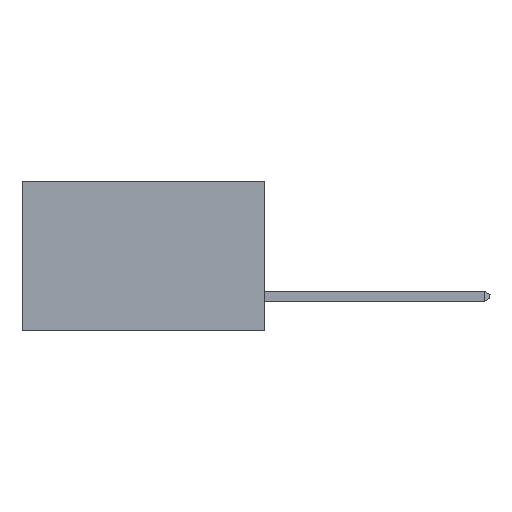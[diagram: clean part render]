
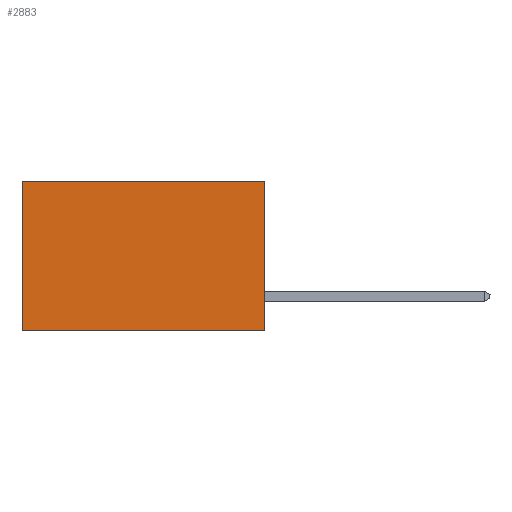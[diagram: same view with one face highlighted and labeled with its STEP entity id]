
A CAD part, left-side view. The second image highlights one B-rep face of the part: STEP entity #2883.
In plain terms, the highlighted planar face has unit normal (-1, 0, 0).
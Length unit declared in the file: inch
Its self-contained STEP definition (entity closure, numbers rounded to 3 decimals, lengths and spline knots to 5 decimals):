
#485 = DIRECTION ( 'NONE',  ( 0., 0., -1. ) ) ;
#1807 = ORIENTED_EDGE ( 'NONE', *, *, #14942, .F. ) ;
#2088 = VERTEX_POINT ( 'NONE', #3233 ) ;
#2535 = CARTESIAN_POINT ( 'NONE',  ( 0.298, 0.6, -0.37 ) ) ;
#2547 = PLANE ( 'NONE',  #7982 ) ;
#2594 = DIRECTION ( 'NONE',  ( 1., 0., 0. ) ) ;
#2863 = LINE ( 'NONE', #11257, #3268 ) ;
#2883 = ADVANCED_FACE ( 'NONE', ( #11976 ), #2547, .F. ) ;
#3084 = CARTESIAN_POINT ( 'NONE',  ( 0.298, 0.6, 0. ) ) ;
#3133 = LINE ( 'NONE', #15592, #11950 ) ;
#3140 = CARTESIAN_POINT ( 'NONE',  ( 0.298, 0.6, 0. ) ) ;
#3233 = CARTESIAN_POINT ( 'NONE',  ( 0.298, 0., 0. ) ) ;
#3268 = VECTOR ( 'NONE', #11429, 39.37008 ) ;
#3695 = DIRECTION ( 'NONE',  ( 0., 1., 0. ) ) ;
#3836 = LINE ( 'NONE', #3084, #4209 ) ;
#4209 = VECTOR ( 'NONE', #485, 39.37008 ) ;
#4692 = DIRECTION ( 'NONE',  ( 0., 0., -1. ) ) ;
#4791 = CARTESIAN_POINT ( 'NONE',  ( 0.298, 0., 0. ) ) ;
#5003 = VERTEX_POINT ( 'NONE', #13782 ) ;
#6920 = ORIENTED_EDGE ( 'NONE', *, *, #10507, .T. ) ;
#7278 = DIRECTION ( 'NONE',  ( 0., 0., -1. ) ) ;
#7982 = AXIS2_PLACEMENT_3D ( 'NONE', #13383, #2594, #7278 ) ;
#9588 = ORIENTED_EDGE ( 'NONE', *, *, #11350, .F. ) ;
#10507 = EDGE_CURVE ( 'NONE', #2088, #15496, #3133, .T. ) ;
#11257 = CARTESIAN_POINT ( 'NONE',  ( 0.298, 0., -0.37 ) ) ;
#11350 = EDGE_CURVE ( 'NONE', #2088, #5003, #14687, .T. ) ;
#11429 = DIRECTION ( 'NONE',  ( 0., 1., 0. ) ) ;
#11950 = VECTOR ( 'NONE', #3695, 39.37008 ) ;
#11976 = FACE_OUTER_BOUND ( 'NONE', #14837, .T. ) ;
#12842 = VERTEX_POINT ( 'NONE', #2535 ) ;
#12987 = VECTOR ( 'NONE', #4692, 39.37008 ) ;
#13383 = CARTESIAN_POINT ( 'NONE',  ( 0.298, 0., 0. ) ) ;
#13750 = ORIENTED_EDGE ( 'NONE', *, *, #14368, .T. ) ;
#13782 = CARTESIAN_POINT ( 'NONE',  ( 0.298, 0., -0.37 ) ) ;
#14368 = EDGE_CURVE ( 'NONE', #15496, #12842, #3836, .T. ) ;
#14687 = LINE ( 'NONE', #4791, #12987 ) ;
#14837 = EDGE_LOOP ( 'NONE', ( #13750, #1807, #9588, #6920 ) ) ;
#14942 = EDGE_CURVE ( 'NONE', #5003, #12842, #2863, .T. ) ;
#15496 = VERTEX_POINT ( 'NONE', #3140 ) ;
#15592 = CARTESIAN_POINT ( 'NONE',  ( 0.298, 0., 0. ) ) ;
